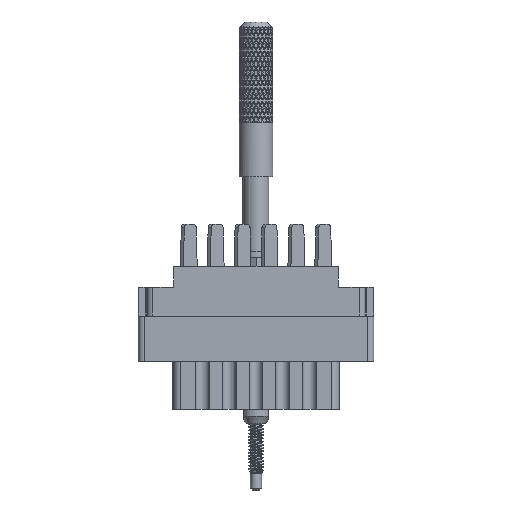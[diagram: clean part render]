
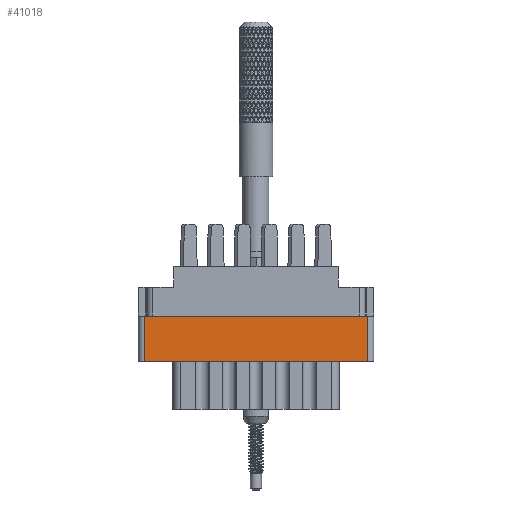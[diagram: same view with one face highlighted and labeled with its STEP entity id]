
A CAD part, front view. The second image highlights one B-rep face of the part: STEP entity #41018.
In plain terms, the highlighted planar face has unit normal (0, -1, 0).
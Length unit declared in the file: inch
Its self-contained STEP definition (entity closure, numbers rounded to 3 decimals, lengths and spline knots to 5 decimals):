
#587 = VECTOR ( 'NONE', #41105, 39.37008 ) ;
#2548 = LINE ( 'NONE', #45150, #163108 ) ;
#3830 = PLANE ( 'NONE',  #80556 ) ;
#4017 = EDGE_CURVE ( 'NONE', #9485, #54782, #2548, .T. ) ;
#5450 = ORIENTED_EDGE ( 'NONE', *, *, #4017, .T. ) ;
#9485 = VERTEX_POINT ( 'NONE', #105560 ) ;
#17786 = CARTESIAN_POINT ( 'NONE',  ( 0.624, -0.343, -0.529 ) ) ;
#31213 = VERTEX_POINT ( 'NONE', #163312 ) ;
#32225 = ORIENTED_EDGE ( 'NONE', *, *, #133559, .F. ) ;
#38035 = ORIENTED_EDGE ( 'NONE', *, *, #60228, .F. ) ;
#41018 = ADVANCED_FACE ( 'NONE', ( #43658 ), #3830, .T. ) ;
#41063 = CARTESIAN_POINT ( 'NONE',  ( -0.624, -0.343, -0.798 ) ) ;
#41105 = DIRECTION ( 'NONE',  ( 1., 0., 0. ) ) ;
#43658 = FACE_OUTER_BOUND ( 'NONE', #168697, .T. ) ;
#45150 = CARTESIAN_POINT ( 'NONE',  ( 0.624, -0.343, -0.798 ) ) ;
#46479 = DIRECTION ( 'NONE',  ( -1., 0., 0. ) ) ;
#54782 = VERTEX_POINT ( 'NONE', #99823 ) ;
#60228 = EDGE_CURVE ( 'NONE', #70482, #54782, #94865, .T. ) ;
#66995 = LINE ( 'NONE', #41063, #172870 ) ;
#70482 = VERTEX_POINT ( 'NONE', #160218 ) ;
#80556 = AXIS2_PLACEMENT_3D ( 'NONE', #141831, #113098, #142752 ) ;
#94865 = LINE ( 'NONE', #152255, #587 ) ;
#99823 = CARTESIAN_POINT ( 'NONE',  ( 0.624, -0.343, -0.277 ) ) ;
#101643 = DIRECTION ( 'NONE',  ( 0., 0., 1. ) ) ;
#105560 = CARTESIAN_POINT ( 'NONE',  ( 0.624, -0.343, -0.529 ) ) ;
#113098 = DIRECTION ( 'NONE',  ( 0., -1., 0. ) ) ;
#115938 = LINE ( 'NONE', #17786, #139287 ) ;
#133559 = EDGE_CURVE ( 'NONE', #9485, #31213, #115938, .T. ) ;
#139287 = VECTOR ( 'NONE', #46479, 39.37008 ) ;
#141831 = CARTESIAN_POINT ( 'NONE',  ( -0.624, -0.343, -0.798 ) ) ;
#142752 = DIRECTION ( 'NONE',  ( 0., 0., -1. ) ) ;
#149647 = EDGE_CURVE ( 'NONE', #31213, #70482, #66995, .T. ) ;
#152255 = CARTESIAN_POINT ( 'NONE',  ( -0.656, -0.343, -0.277 ) ) ;
#160218 = CARTESIAN_POINT ( 'NONE',  ( -0.624, -0.343, -0.277 ) ) ;
#163108 = VECTOR ( 'NONE', #101643, 39.37008 ) ;
#163312 = CARTESIAN_POINT ( 'NONE',  ( -0.624, -0.343, -0.529 ) ) ;
#167002 = DIRECTION ( 'NONE',  ( 0., 0., 1. ) ) ;
#168697 = EDGE_LOOP ( 'NONE', ( #171735, #32225, #5450, #38035 ) ) ;
#171735 = ORIENTED_EDGE ( 'NONE', *, *, #149647, .F. ) ;
#172870 = VECTOR ( 'NONE', #167002, 39.37008 ) ;
